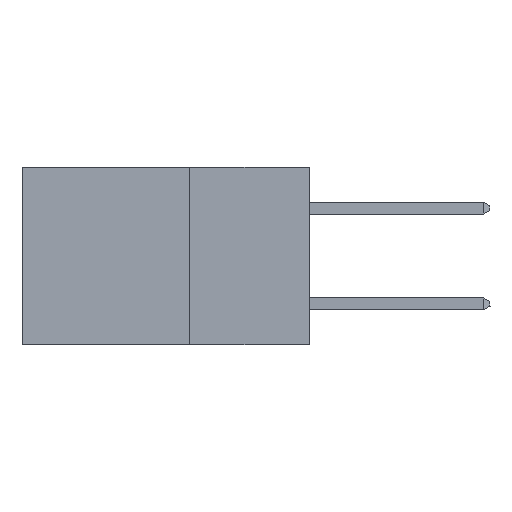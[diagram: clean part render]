
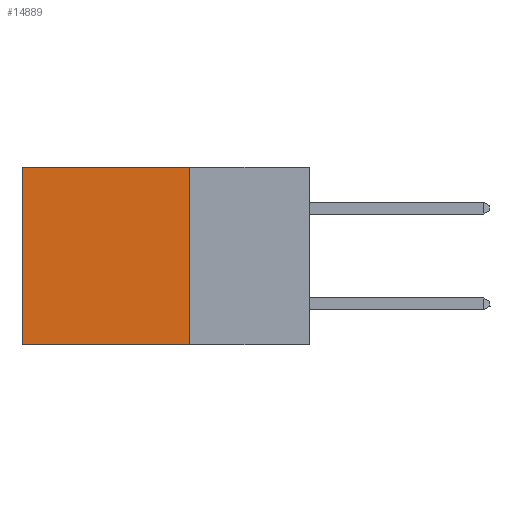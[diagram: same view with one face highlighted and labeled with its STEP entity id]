
A CAD part, left-side view. The second image highlights one B-rep face of the part: STEP entity #14889.
In plain terms, the highlighted planar face has unit normal (-1, 0, 0).
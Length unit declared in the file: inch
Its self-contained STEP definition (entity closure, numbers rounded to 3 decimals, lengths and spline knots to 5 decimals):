
#773 = ORIENTED_EDGE ( 'NONE', *, *, #1156, .F. ) ;
#1156 = EDGE_CURVE ( 'NONE', #2309, #17415, #9027, .T. ) ;
#1219 = CARTESIAN_POINT ( 'NONE',  ( 0.2875, 0.25, 0. ) ) ;
#1688 = EDGE_CURVE ( 'NONE', #11439, #17415, #7386, .T. ) ;
#2125 = FACE_OUTER_BOUND ( 'NONE', #19213, .T. ) ;
#2309 = VERTEX_POINT ( 'NONE', #19462 ) ;
#3141 = ORIENTED_EDGE ( 'NONE', *, *, #15475, .F. ) ;
#3952 = CARTESIAN_POINT ( 'NONE',  ( 0.2875, 0.25, 0. ) ) ;
#4495 = CARTESIAN_POINT ( 'NONE',  ( 0.2875, 0.25, 0. ) ) ;
#5178 = AXIS2_PLACEMENT_3D ( 'NONE', #3952, #10328, #18635 ) ;
#5193 = LINE ( 'NONE', #6488, #12084 ) ;
#5231 = VECTOR ( 'NONE', #20684, 39.37008 ) ;
#5742 = DIRECTION ( 'NONE',  ( 0., 1., 0. ) ) ;
#5878 = VECTOR ( 'NONE', #5742, 39.37008 ) ;
#6297 = CARTESIAN_POINT ( 'NONE',  ( 0.2875, 0.6, -0.37 ) ) ;
#6488 = CARTESIAN_POINT ( 'NONE',  ( 0.2875, 0.25, 0. ) ) ;
#7386 = LINE ( 'NONE', #7700, #5231 ) ;
#7583 = VECTOR ( 'NONE', #14212, 39.37008 ) ;
#7700 = CARTESIAN_POINT ( 'NONE',  ( 0.2875, 0.6, 0. ) ) ;
#8027 = ORIENTED_EDGE ( 'NONE', *, *, #20218, .T. ) ;
#9027 = LINE ( 'NONE', #15532, #5878 ) ;
#10328 = DIRECTION ( 'NONE',  ( 1., 0., 0. ) ) ;
#11439 = VERTEX_POINT ( 'NONE', #11872 ) ;
#11872 = CARTESIAN_POINT ( 'NONE',  ( 0.2875, 0.6, 0. ) ) ;
#12084 = VECTOR ( 'NONE', #17866, 39.37008 ) ;
#14212 = DIRECTION ( 'NONE',  ( 0., 0., -1. ) ) ;
#14351 = ORIENTED_EDGE ( 'NONE', *, *, #1688, .T. ) ;
#14889 = ADVANCED_FACE ( 'NONE', ( #2125 ), #16837, .F. ) ;
#15475 = EDGE_CURVE ( 'NONE', #20861, #2309, #15831, .T. ) ;
#15532 = CARTESIAN_POINT ( 'NONE',  ( 0.2875, 0.25, -0.37 ) ) ;
#15831 = LINE ( 'NONE', #1219, #7583 ) ;
#16837 = PLANE ( 'NONE',  #5178 ) ;
#17415 = VERTEX_POINT ( 'NONE', #6297 ) ;
#17866 = DIRECTION ( 'NONE',  ( 0., 1., 0. ) ) ;
#18635 = DIRECTION ( 'NONE',  ( 0., 0., -1. ) ) ;
#19213 = EDGE_LOOP ( 'NONE', ( #14351, #773, #3141, #8027 ) ) ;
#19462 = CARTESIAN_POINT ( 'NONE',  ( 0.2875, 0.25, -0.37 ) ) ;
#20218 = EDGE_CURVE ( 'NONE', #20861, #11439, #5193, .T. ) ;
#20684 = DIRECTION ( 'NONE',  ( 0., 0., -1. ) ) ;
#20861 = VERTEX_POINT ( 'NONE', #4495 ) ;
